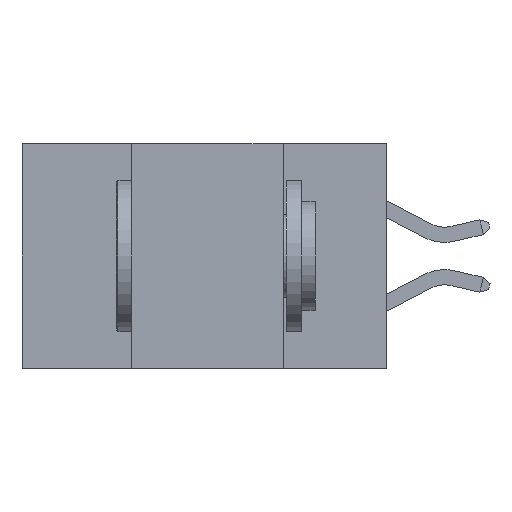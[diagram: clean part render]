
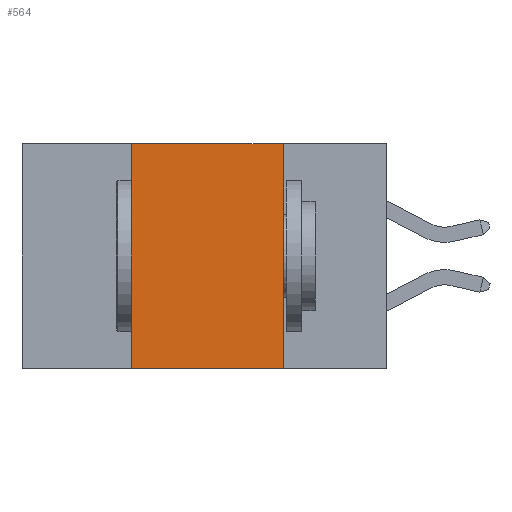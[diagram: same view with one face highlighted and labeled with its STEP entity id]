
A CAD part, left-side view. The second image highlights one B-rep face of the part: STEP entity #564.
In plain terms, the highlighted planar face has unit normal (-1, 0, 0).
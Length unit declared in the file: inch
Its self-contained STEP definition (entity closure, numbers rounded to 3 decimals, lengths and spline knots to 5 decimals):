
#227 = FACE_OUTER_BOUND ( 'NONE', #10962, .T. ) ;
#339 = VECTOR ( 'NONE', #884, 39.37008 ) ;
#564 = ADVANCED_FACE ( 'NONE', ( #227 ), #8573, .F. ) ;
#608 = EDGE_CURVE ( 'NONE', #3366, #1152, #7789, .T. ) ;
#686 = ORIENTED_EDGE ( 'NONE', *, *, #608, .F. ) ;
#884 = DIRECTION ( 'NONE',  ( 0., 0., 1. ) ) ;
#1152 = VERTEX_POINT ( 'NONE', #4277 ) ;
#1659 = DIRECTION ( 'NONE',  ( 1., 0., 0. ) ) ;
#2030 = EDGE_CURVE ( 'NONE', #3822, #5578, #9478, .T. ) ;
#2280 = EDGE_CURVE ( 'NONE', #3822, #3366, #8077, .T. ) ;
#3366 = VERTEX_POINT ( 'NONE', #6620 ) ;
#3519 = DIRECTION ( 'NONE',  ( 0., 0., -1. ) ) ;
#3822 = VERTEX_POINT ( 'NONE', #8206 ) ;
#4111 = CARTESIAN_POINT ( 'NONE',  ( 0., 0.6, 0. ) ) ;
#4274 = DIRECTION ( 'NONE',  ( 0., -1., 0. ) ) ;
#4277 = CARTESIAN_POINT ( 'NONE',  ( 0., 0.17, 0. ) ) ;
#4815 = LINE ( 'NONE', #7100, #7901 ) ;
#5578 = VERTEX_POINT ( 'NONE', #10585 ) ;
#6238 = ORIENTED_EDGE ( 'NONE', *, *, #2280, .F. ) ;
#6620 = CARTESIAN_POINT ( 'NONE',  ( 0., 0.42, 0. ) ) ;
#7013 = VECTOR ( 'NONE', #7937, 39.37008 ) ;
#7100 = CARTESIAN_POINT ( 'NONE',  ( 0., 0.17, 0. ) ) ;
#7789 = LINE ( 'NONE', #9642, #12061 ) ;
#7901 = VECTOR ( 'NONE', #3519, 39.37008 ) ;
#7937 = DIRECTION ( 'NONE',  ( 0., -1., 0. ) ) ;
#8077 = LINE ( 'NONE', #12439, #339 ) ;
#8206 = CARTESIAN_POINT ( 'NONE',  ( 0., 0.42, -0.37 ) ) ;
#8573 = PLANE ( 'NONE',  #14222 ) ;
#9478 = LINE ( 'NONE', #13673, #7013 ) ;
#9507 = ORIENTED_EDGE ( 'NONE', *, *, #2030, .T. ) ;
#9642 = CARTESIAN_POINT ( 'NONE',  ( 0., 0.6, 0. ) ) ;
#9691 = DIRECTION ( 'NONE',  ( 0., 0., -1. ) ) ;
#10585 = CARTESIAN_POINT ( 'NONE',  ( 0., 0.17, -0.37 ) ) ;
#10962 = EDGE_LOOP ( 'NONE', ( #11444, #686, #6238, #9507 ) ) ;
#11444 = ORIENTED_EDGE ( 'NONE', *, *, #11619, .F. ) ;
#11619 = EDGE_CURVE ( 'NONE', #1152, #5578, #4815, .T. ) ;
#12061 = VECTOR ( 'NONE', #4274, 39.37008 ) ;
#12439 = CARTESIAN_POINT ( 'NONE',  ( 0., 0.42, 0. ) ) ;
#13673 = CARTESIAN_POINT ( 'NONE',  ( 0., 0.6, -0.37 ) ) ;
#14222 = AXIS2_PLACEMENT_3D ( 'NONE', #4111, #1659, #9691 ) ;
